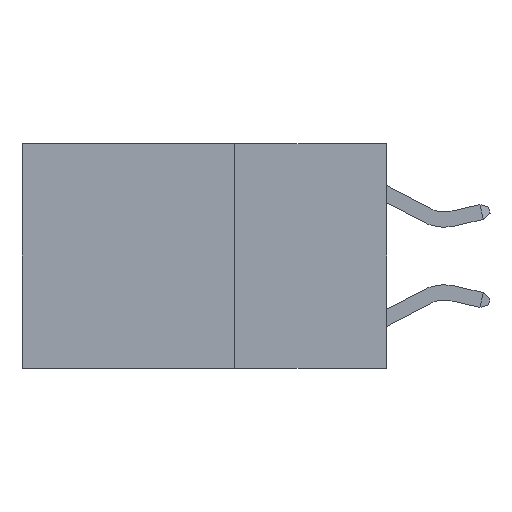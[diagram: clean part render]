
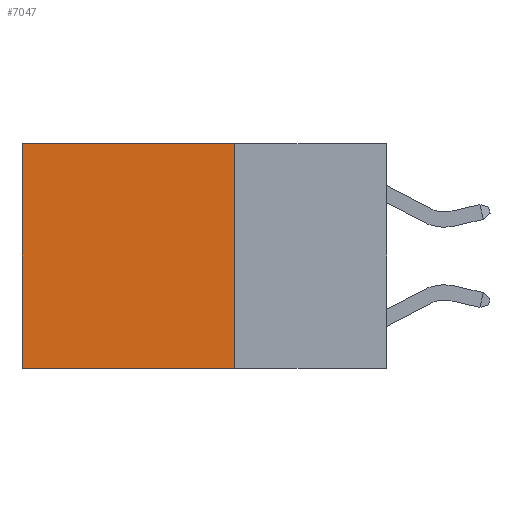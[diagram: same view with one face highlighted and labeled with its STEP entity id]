
A CAD part, left-side view. The second image highlights one B-rep face of the part: STEP entity #7047.
In plain terms, the highlighted planar face has unit normal (-1, 0, 0).
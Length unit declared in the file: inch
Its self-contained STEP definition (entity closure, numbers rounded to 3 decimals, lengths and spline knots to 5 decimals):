
#173 = ORIENTED_EDGE ( 'NONE', *, *, #7194, .F. ) ;
#537 = VERTEX_POINT ( 'NONE', #2305 ) ;
#750 = LINE ( 'NONE', #5159, #4439 ) ;
#891 = CARTESIAN_POINT ( 'NONE',  ( 0.2625, 0.6, 0. ) ) ;
#1261 = EDGE_CURVE ( 'NONE', #6647, #6621, #1769, .T. ) ;
#1769 = LINE ( 'NONE', #891, #4916 ) ;
#1871 = DIRECTION ( 'NONE',  ( 0., 0., -1. ) ) ;
#2305 = CARTESIAN_POINT ( 'NONE',  ( 0.2625, 0.25, -0.37 ) ) ;
#2353 = CARTESIAN_POINT ( 'NONE',  ( 0.2625, 0.25, 0. ) ) ;
#2463 = LINE ( 'NONE', #5938, #3693 ) ;
#3098 = DIRECTION ( 'NONE',  ( 0., 0., -1. ) ) ;
#3693 = VECTOR ( 'NONE', #1871, 39.37008 ) ;
#3944 = FACE_OUTER_BOUND ( 'NONE', #9195, .T. ) ;
#4439 = VECTOR ( 'NONE', #9440, 39.37008 ) ;
#4638 = CARTESIAN_POINT ( 'NONE',  ( 0.2625, 0.6, -0.37 ) ) ;
#4916 = VECTOR ( 'NONE', #7000, 39.37008 ) ;
#5159 = CARTESIAN_POINT ( 'NONE',  ( 0.2625, 0.25, -0.37 ) ) ;
#5423 = CARTESIAN_POINT ( 'NONE',  ( 0.2625, 0.25, 0. ) ) ;
#5519 = AXIS2_PLACEMENT_3D ( 'NONE', #5423, #5818, #3098 ) ;
#5818 = DIRECTION ( 'NONE',  ( 1., 0., 0. ) ) ;
#5823 = ORIENTED_EDGE ( 'NONE', *, *, #1261, .T. ) ;
#5938 = CARTESIAN_POINT ( 'NONE',  ( 0.2625, 0.25, 0. ) ) ;
#6355 = ORIENTED_EDGE ( 'NONE', *, *, #9182, .T. ) ;
#6621 = VERTEX_POINT ( 'NONE', #4638 ) ;
#6647 = VERTEX_POINT ( 'NONE', #10758 ) ;
#7000 = DIRECTION ( 'NONE',  ( 0., 0., -1. ) ) ;
#7047 = ADVANCED_FACE ( 'NONE', ( #3944 ), #7386, .F. ) ;
#7194 = EDGE_CURVE ( 'NONE', #8600, #537, #2463, .T. ) ;
#7386 = PLANE ( 'NONE',  #5519 ) ;
#7710 = VECTOR ( 'NONE', #9239, 39.37008 ) ;
#8183 = EDGE_CURVE ( 'NONE', #537, #6621, #750, .T. ) ;
#8600 = VERTEX_POINT ( 'NONE', #10030 ) ;
#9182 = EDGE_CURVE ( 'NONE', #8600, #6647, #10128, .T. ) ;
#9195 = EDGE_LOOP ( 'NONE', ( #5823, #10052, #173, #6355 ) ) ;
#9239 = DIRECTION ( 'NONE',  ( 0., 1., 0. ) ) ;
#9440 = DIRECTION ( 'NONE',  ( 0., 1., 0. ) ) ;
#10030 = CARTESIAN_POINT ( 'NONE',  ( 0.2625, 0.25, 0. ) ) ;
#10052 = ORIENTED_EDGE ( 'NONE', *, *, #8183, .F. ) ;
#10128 = LINE ( 'NONE', #2353, #7710 ) ;
#10758 = CARTESIAN_POINT ( 'NONE',  ( 0.2625, 0.6, 0. ) ) ;
